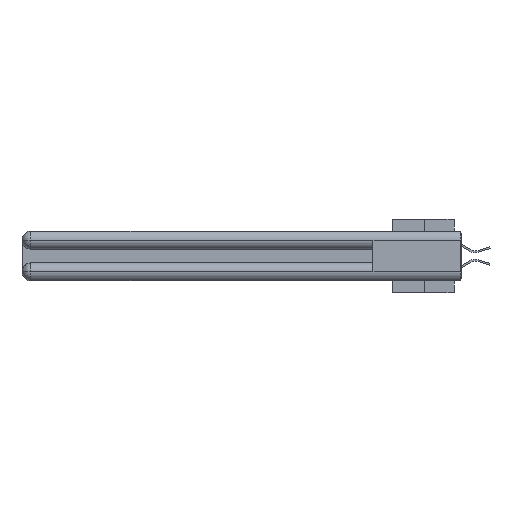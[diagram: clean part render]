
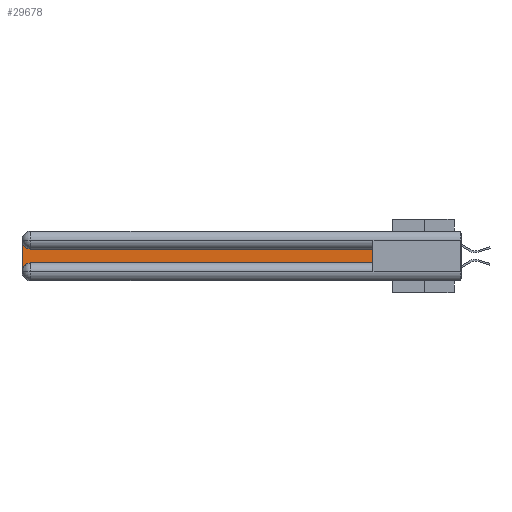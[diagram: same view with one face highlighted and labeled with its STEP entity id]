
A CAD part, left-side view. The second image highlights one B-rep face of the part: STEP entity #29678.
In plain terms, the highlighted planar face has unit normal (-1, 0, 0).
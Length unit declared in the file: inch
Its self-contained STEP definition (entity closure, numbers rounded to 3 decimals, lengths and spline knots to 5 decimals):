
#492 = CARTESIAN_POINT ( 'NONE',  ( 0.075, 2.94, -0.2175 ) ) ;
#933 = LINE ( 'NONE', #7608, #3085 ) ;
#3019 = ORIENTED_EDGE ( 'NONE', *, *, #20177, .T. ) ;
#3085 = VECTOR ( 'NONE', #18732, 39.37008 ) ;
#4370 = VECTOR ( 'NONE', #25189, 39.37008 ) ;
#4433 = EDGE_CURVE ( 'NONE', #29999, #23917, #21083, .T. ) ;
#4748 = VERTEX_POINT ( 'NONE', #28136 ) ;
#4899 = DIRECTION ( 'NONE',  ( 0., 0., -1. ) ) ;
#5462 = ORIENTED_EDGE ( 'NONE', *, *, #20739, .T. ) ;
#5762 = DIRECTION ( 'NONE',  ( 0., -1., 0. ) ) ;
#6246 = CARTESIAN_POINT ( 'NONE',  ( 0.075, 3., -0.0625 ) ) ;
#7515 = ORIENTED_EDGE ( 'NONE', *, *, #34278, .T. ) ;
#7608 = CARTESIAN_POINT ( 'NONE',  ( 0.075, 0.6, -0.2175 ) ) ;
#8342 = CARTESIAN_POINT ( 'NONE',  ( 0.075, 0.6, -0.2175 ) ) ;
#8855 = AXIS2_PLACEMENT_3D ( 'NONE', #13340, #32081, #15996 ) ;
#10985 = VERTEX_POINT ( 'NONE', #19479 ) ;
#11898 = DIRECTION ( 'NONE',  ( 1., 0., 0. ) ) ;
#13340 = CARTESIAN_POINT ( 'NONE',  ( 0.075, 2.94, -0.2775 ) ) ;
#13354 = LINE ( 'NONE', #28786, #26768 ) ;
#14566 = DIRECTION ( 'NONE',  ( 0., 0., -1. ) ) ;
#15477 = ORIENTED_EDGE ( 'NONE', *, *, #28052, .T. ) ;
#15678 = CIRCLE ( 'NONE', #8855, 0.06 ) ;
#15858 = PLANE ( 'NONE',  #24868 ) ;
#15996 = DIRECTION ( 'NONE',  ( 0., 0., -1. ) ) ;
#16163 = CARTESIAN_POINT ( 'NONE',  ( 0.075, 0.6, -0.2175 ) ) ;
#16169 = CIRCLE ( 'NONE', #18432, 0.06 ) ;
#16439 = VERTEX_POINT ( 'NONE', #8342 ) ;
#18432 = AXIS2_PLACEMENT_3D ( 'NONE', #19814, #11898, #14566 ) ;
#18732 = DIRECTION ( 'NONE',  ( 0., 0., 1. ) ) ;
#19131 = VECTOR ( 'NONE', #5762, 39.37008 ) ;
#19479 = CARTESIAN_POINT ( 'NONE',  ( 0.075, 0.6, -0.1225 ) ) ;
#19814 = CARTESIAN_POINT ( 'NONE',  ( 0.075, 2.94, -0.0625 ) ) ;
#19961 = LINE ( 'NONE', #16163, #19131 ) ;
#20177 = EDGE_CURVE ( 'NONE', #23917, #29819, #15678, .T. ) ;
#20739 = EDGE_CURVE ( 'NONE', #16439, #10985, #933, .T. ) ;
#21083 = LINE ( 'NONE', #22588, #4370 ) ;
#21127 = DIRECTION ( 'NONE',  ( 1., 0., 0. ) ) ;
#22588 = CARTESIAN_POINT ( 'NONE',  ( 0.075, 3., -0.2175 ) ) ;
#23917 = VERTEX_POINT ( 'NONE', #24697 ) ;
#24289 = ORIENTED_EDGE ( 'NONE', *, *, #33521, .T. ) ;
#24536 = ORIENTED_EDGE ( 'NONE', *, *, #4433, .T. ) ;
#24697 = CARTESIAN_POINT ( 'NONE',  ( 0.075, 3., -0.2775 ) ) ;
#24868 = AXIS2_PLACEMENT_3D ( 'NONE', #31699, #21127, #4899 ) ;
#24980 = FACE_OUTER_BOUND ( 'NONE', #31379, .T. ) ;
#25189 = DIRECTION ( 'NONE',  ( 0., 0., -1. ) ) ;
#26768 = VECTOR ( 'NONE', #33919, 39.37008 ) ;
#28052 = EDGE_CURVE ( 'NONE', #4748, #29999, #16169, .T. ) ;
#28136 = CARTESIAN_POINT ( 'NONE',  ( 0.075, 2.94, -0.1225 ) ) ;
#28786 = CARTESIAN_POINT ( 'NONE',  ( 0.075, 0.6, -0.1225 ) ) ;
#29678 = ADVANCED_FACE ( 'NONE', ( #24980 ), #15858, .F. ) ;
#29819 = VERTEX_POINT ( 'NONE', #492 ) ;
#29999 = VERTEX_POINT ( 'NONE', #6246 ) ;
#31379 = EDGE_LOOP ( 'NONE', ( #24289, #15477, #24536, #3019, #7515, #5462 ) ) ;
#31699 = CARTESIAN_POINT ( 'NONE',  ( 0.075, 3., -0.1225 ) ) ;
#32081 = DIRECTION ( 'NONE',  ( 1., 0., 0. ) ) ;
#33521 = EDGE_CURVE ( 'NONE', #10985, #4748, #13354, .T. ) ;
#33919 = DIRECTION ( 'NONE',  ( 0., 1., 0. ) ) ;
#34278 = EDGE_CURVE ( 'NONE', #29819, #16439, #19961, .T. ) ;
